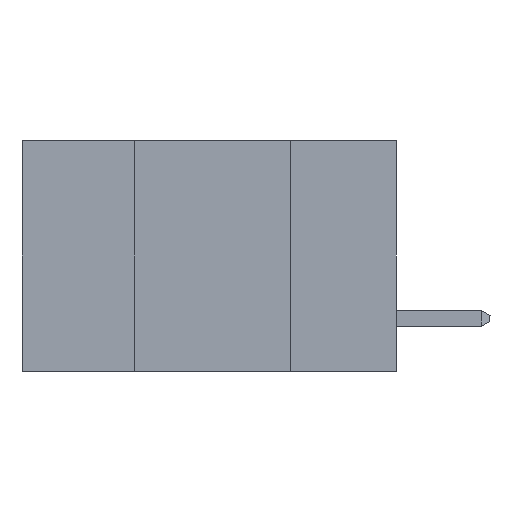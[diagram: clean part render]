
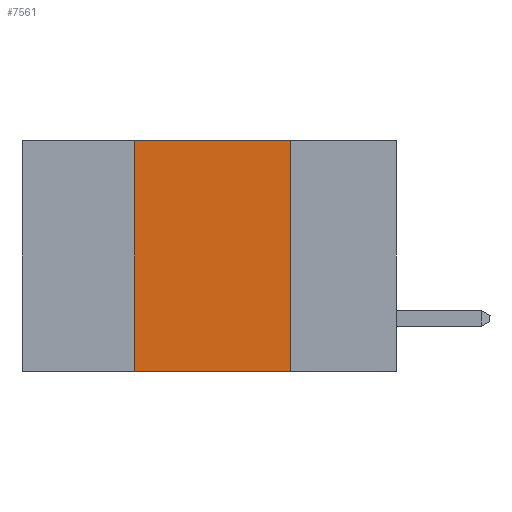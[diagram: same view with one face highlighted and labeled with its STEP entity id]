
A CAD part, left-side view. The second image highlights one B-rep face of the part: STEP entity #7561.
In plain terms, the highlighted planar face has unit normal (-1, 0, 0).
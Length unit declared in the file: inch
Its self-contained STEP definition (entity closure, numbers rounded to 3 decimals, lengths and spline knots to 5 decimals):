
#960 = DIRECTION ( 'NONE',  ( 0., 0., -1. ) ) ;
#1760 = VERTEX_POINT ( 'NONE', #2897 ) ;
#2198 = DIRECTION ( 'NONE',  ( 1., 0., 0. ) ) ;
#2702 = VECTOR ( 'NONE', #12981, 39.37008 ) ;
#2897 = CARTESIAN_POINT ( 'NONE',  ( 0., 0.42, 0. ) ) ;
#3060 = EDGE_CURVE ( 'NONE', #14741, #5737, #6842, .T. ) ;
#3721 = EDGE_LOOP ( 'NONE', ( #10044, #10906, #15210, #9445 ) ) ;
#5125 = EDGE_CURVE ( 'NONE', #13061, #1760, #8336, .T. ) ;
#5737 = VERTEX_POINT ( 'NONE', #10147 ) ;
#6010 = AXIS2_PLACEMENT_3D ( 'NONE', #12906, #2198, #960 ) ;
#6039 = EDGE_CURVE ( 'NONE', #13061, #5737, #10979, .T. ) ;
#6441 = CARTESIAN_POINT ( 'NONE',  ( 0., 0.6, -0.37 ) ) ;
#6538 = VECTOR ( 'NONE', #13373, 39.37008 ) ;
#6842 = LINE ( 'NONE', #13678, #14799 ) ;
#7561 = ADVANCED_FACE ( 'NONE', ( #12746 ), #15207, .F. ) ;
#8336 = LINE ( 'NONE', #10653, #15133 ) ;
#9445 = ORIENTED_EDGE ( 'NONE', *, *, #6039, .T. ) ;
#10044 = ORIENTED_EDGE ( 'NONE', *, *, #3060, .F. ) ;
#10147 = CARTESIAN_POINT ( 'NONE',  ( 0., 0.17, -0.37 ) ) ;
#10534 = CARTESIAN_POINT ( 'NONE',  ( 0., 0.42, -0.37 ) ) ;
#10653 = CARTESIAN_POINT ( 'NONE',  ( 0., 0.42, -0.37 ) ) ;
#10738 = CARTESIAN_POINT ( 'NONE',  ( 0., 0.6, 0. ) ) ;
#10906 = ORIENTED_EDGE ( 'NONE', *, *, #12147, .F. ) ;
#10979 = LINE ( 'NONE', #6441, #6538 ) ;
#11525 = DIRECTION ( 'NONE',  ( 0., 0., -1. ) ) ;
#12147 = EDGE_CURVE ( 'NONE', #1760, #14741, #12755, .T. ) ;
#12555 = CARTESIAN_POINT ( 'NONE',  ( 0., 0.17, 0. ) ) ;
#12746 = FACE_OUTER_BOUND ( 'NONE', #3721, .T. ) ;
#12755 = LINE ( 'NONE', #10738, #2702 ) ;
#12906 = CARTESIAN_POINT ( 'NONE',  ( 0., 0.6, 0. ) ) ;
#12981 = DIRECTION ( 'NONE',  ( 0., -1., 0. ) ) ;
#13035 = DIRECTION ( 'NONE',  ( 0., 0., 1. ) ) ;
#13061 = VERTEX_POINT ( 'NONE', #10534 ) ;
#13373 = DIRECTION ( 'NONE',  ( 0., -1., 0. ) ) ;
#13678 = CARTESIAN_POINT ( 'NONE',  ( 0., 0.17, -0.37 ) ) ;
#14741 = VERTEX_POINT ( 'NONE', #12555 ) ;
#14799 = VECTOR ( 'NONE', #11525, 39.37008 ) ;
#15133 = VECTOR ( 'NONE', #13035, 39.37008 ) ;
#15207 = PLANE ( 'NONE',  #6010 ) ;
#15210 = ORIENTED_EDGE ( 'NONE', *, *, #5125, .F. ) ;
